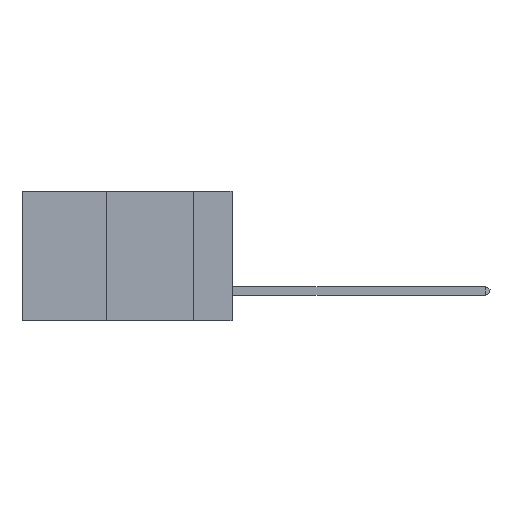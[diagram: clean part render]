
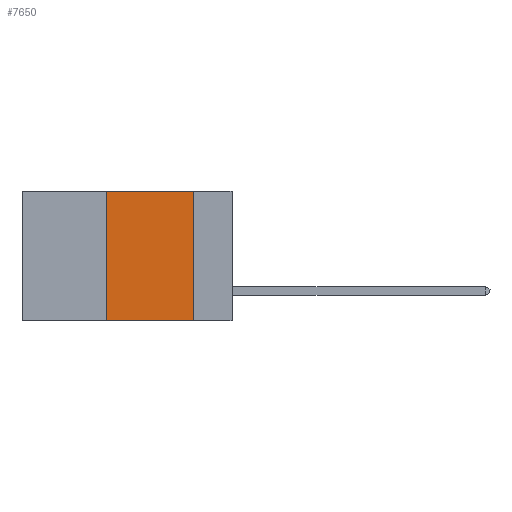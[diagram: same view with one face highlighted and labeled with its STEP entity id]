
A CAD part, left-side view. The second image highlights one B-rep face of the part: STEP entity #7650.
In plain terms, the highlighted planar face has unit normal (-1, 0, 0).
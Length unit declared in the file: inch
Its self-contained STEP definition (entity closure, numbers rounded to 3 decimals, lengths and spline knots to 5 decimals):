
#178 = LINE ( 'NONE', #4199, #4902 ) ;
#361 = VERTEX_POINT ( 'NONE', #11981 ) ;
#619 = CARTESIAN_POINT ( 'NONE',  ( 0., 0.11, 0. ) ) ;
#786 = DIRECTION ( 'NONE',  ( 0., 0., -1. ) ) ;
#1008 = DIRECTION ( 'NONE',  ( 0., -1., 0. ) ) ;
#1419 = CARTESIAN_POINT ( 'NONE',  ( 0., 0.6, -0.37 ) ) ;
#1602 = EDGE_LOOP ( 'NONE', ( #3429, #5994, #10023, #1889 ) ) ;
#1724 = LINE ( 'NONE', #11725, #12869 ) ;
#1837 = CARTESIAN_POINT ( 'NONE',  ( 0., 0.6, 0. ) ) ;
#1889 = ORIENTED_EDGE ( 'NONE', *, *, #12165, .T. ) ;
#3243 = LINE ( 'NONE', #3376, #11791 ) ;
#3376 = CARTESIAN_POINT ( 'NONE',  ( 0., 0.11, 0. ) ) ;
#3429 = ORIENTED_EDGE ( 'NONE', *, *, #5725, .F. ) ;
#3822 = DIRECTION ( 'NONE',  ( 1., 0., 0. ) ) ;
#3902 = VERTEX_POINT ( 'NONE', #9017 ) ;
#4199 = CARTESIAN_POINT ( 'NONE',  ( 0., 0.36, 0. ) ) ;
#4902 = VECTOR ( 'NONE', #12231, 39.37008 ) ;
#5403 = VERTEX_POINT ( 'NONE', #619 ) ;
#5725 = EDGE_CURVE ( 'NONE', #5403, #361, #3243, .T. ) ;
#5737 = AXIS2_PLACEMENT_3D ( 'NONE', #1837, #3822, #786 ) ;
#5889 = EDGE_CURVE ( 'NONE', #3902, #5403, #1724, .T. ) ;
#5994 = ORIENTED_EDGE ( 'NONE', *, *, #5889, .F. ) ;
#6135 = DIRECTION ( 'NONE',  ( 0., 0., -1. ) ) ;
#6205 = LINE ( 'NONE', #1419, #7283 ) ;
#7283 = VECTOR ( 'NONE', #12146, 39.37008 ) ;
#7650 = ADVANCED_FACE ( 'NONE', ( #10728 ), #12844, .F. ) ;
#7776 = CARTESIAN_POINT ( 'NONE',  ( 0., 0.36, -0.37 ) ) ;
#7823 = EDGE_CURVE ( 'NONE', #8941, #3902, #178, .T. ) ;
#8941 = VERTEX_POINT ( 'NONE', #7776 ) ;
#9017 = CARTESIAN_POINT ( 'NONE',  ( 0., 0.36, 0. ) ) ;
#10023 = ORIENTED_EDGE ( 'NONE', *, *, #7823, .F. ) ;
#10728 = FACE_OUTER_BOUND ( 'NONE', #1602, .T. ) ;
#11725 = CARTESIAN_POINT ( 'NONE',  ( 0., 0.6, 0. ) ) ;
#11791 = VECTOR ( 'NONE', #6135, 39.37008 ) ;
#11981 = CARTESIAN_POINT ( 'NONE',  ( 0., 0.11, -0.37 ) ) ;
#12146 = DIRECTION ( 'NONE',  ( 0., -1., 0. ) ) ;
#12165 = EDGE_CURVE ( 'NONE', #8941, #361, #6205, .T. ) ;
#12231 = DIRECTION ( 'NONE',  ( 0., 0., 1. ) ) ;
#12844 = PLANE ( 'NONE',  #5737 ) ;
#12869 = VECTOR ( 'NONE', #1008, 39.37008 ) ;
